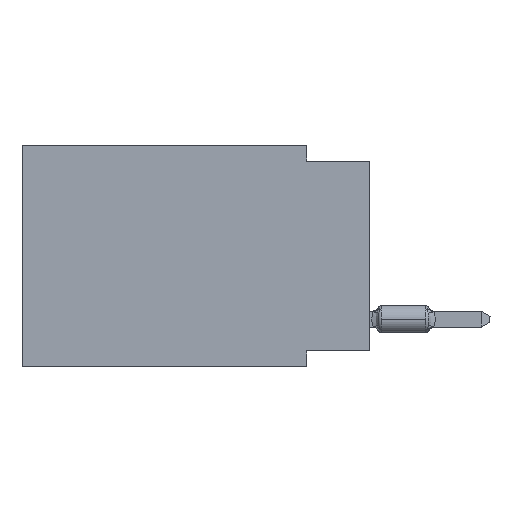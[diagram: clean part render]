
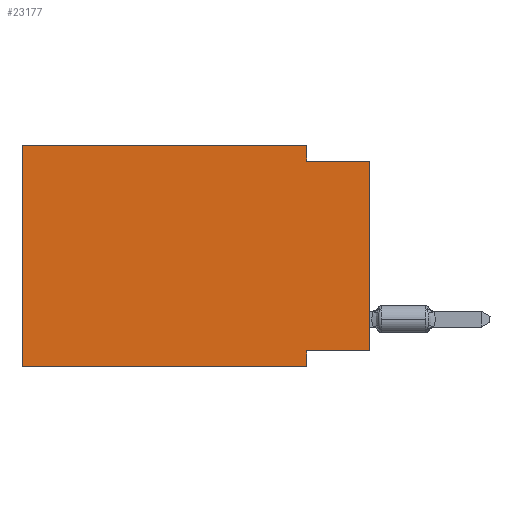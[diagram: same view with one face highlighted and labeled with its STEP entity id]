
A CAD part, left-side view. The second image highlights one B-rep face of the part: STEP entity #23177.
In plain terms, the highlighted planar face has unit normal (-1, 0, 0).
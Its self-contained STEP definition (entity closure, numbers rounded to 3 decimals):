
#3255 = DIRECTION ( 'NONE',  ( 1., 0., 0. ) ) ;
#3446 = VECTOR ( 'NONE', #14922, 1000. ) ;
#4065 = VERTEX_POINT ( 'NONE', #30810 ) ;
#4188 = VERTEX_POINT ( 'NONE', #8669 ) ;
#4518 = EDGE_CURVE ( 'NONE', #20491, #4188, #23478, .T. ) ;
#4533 = ORIENTED_EDGE ( 'NONE', *, *, #8984, .F. ) ;
#5095 = CARTESIAN_POINT ( 'NONE',  ( 0., 2.54, 0. ) ) ;
#5381 = CARTESIAN_POINT ( 'NONE',  ( 0., 13.97, 0. ) ) ;
#5508 = EDGE_CURVE ( 'NONE', #20491, #24755, #15888, .T. ) ;
#6417 = ORIENTED_EDGE ( 'NONE', *, *, #20811, .F. ) ;
#6539 = LINE ( 'NONE', #8978, #17832 ) ;
#6887 = ORIENTED_EDGE ( 'NONE', *, *, #11099, .T. ) ;
#6951 = EDGE_CURVE ( 'NONE', #24755, #10226, #9749, .T. ) ;
#7916 = EDGE_LOOP ( 'NONE', ( #22343, #30925, #11296, #4533, #6417, #6887, #31349, #20226 ) ) ;
#8182 = VECTOR ( 'NONE', #29321, 1000. ) ;
#8552 = VECTOR ( 'NONE', #33513, 1000. ) ;
#8659 = PLANE ( 'NONE',  #29451 ) ;
#8669 = CARTESIAN_POINT ( 'NONE',  ( 0., 0., -0.635 ) ) ;
#8978 = CARTESIAN_POINT ( 'NONE',  ( 0., 13.97, 0. ) ) ;
#8984 = EDGE_CURVE ( 'NONE', #32843, #20707, #32908, .T. ) ;
#9140 = EDGE_CURVE ( 'NONE', #4065, #4188, #30639, .T. ) ;
#9142 = VECTOR ( 'NONE', #15730, 1000. ) ;
#9749 = LINE ( 'NONE', #17945, #20324 ) ;
#10226 = VERTEX_POINT ( 'NONE', #16858 ) ;
#11099 = EDGE_CURVE ( 'NONE', #18466, #10226, #22703, .T. ) ;
#11296 = ORIENTED_EDGE ( 'NONE', *, *, #29015, .F. ) ;
#12833 = DIRECTION ( 'NONE',  ( 0., 0., 1. ) ) ;
#13177 = CARTESIAN_POINT ( 'NONE',  ( 0., 13.97, -8.89 ) ) ;
#13541 = CARTESIAN_POINT ( 'NONE',  ( 0., 2.54, 0. ) ) ;
#14564 = DIRECTION ( 'NONE',  ( 0., 0., 1. ) ) ;
#14922 = DIRECTION ( 'NONE',  ( 0., -1., 0. ) ) ;
#15149 = VECTOR ( 'NONE', #18788, 1000. ) ;
#15282 = CARTESIAN_POINT ( 'NONE',  ( 0., 0., 0. ) ) ;
#15730 = DIRECTION ( 'NONE',  ( 0., 0., -1. ) ) ;
#15888 = LINE ( 'NONE', #21978, #8182 ) ;
#16858 = CARTESIAN_POINT ( 'NONE',  ( 0., 2.54, -8.89 ) ) ;
#17832 = VECTOR ( 'NONE', #14564, 1000. ) ;
#17945 = CARTESIAN_POINT ( 'NONE',  ( 0., 2.54, -8.89 ) ) ;
#18466 = VERTEX_POINT ( 'NONE', #13177 ) ;
#18788 = DIRECTION ( 'NONE',  ( 0., -1., 0. ) ) ;
#20226 = ORIENTED_EDGE ( 'NONE', *, *, #5508, .F. ) ;
#20324 = VECTOR ( 'NONE', #26322, 1000. ) ;
#20491 = VERTEX_POINT ( 'NONE', #28205 ) ;
#20707 = VERTEX_POINT ( 'NONE', #13541 ) ;
#20811 = EDGE_CURVE ( 'NONE', #18466, #32843, #6539, .T. ) ;
#21978 = CARTESIAN_POINT ( 'NONE',  ( 0., 0., -8.255 ) ) ;
#22343 = ORIENTED_EDGE ( 'NONE', *, *, #4518, .T. ) ;
#22703 = LINE ( 'NONE', #30901, #8552 ) ;
#23177 = ADVANCED_FACE ( 'NONE', ( #32569 ), #8659, .F. ) ;
#23478 = LINE ( 'NONE', #15282, #26474 ) ;
#23912 = CARTESIAN_POINT ( 'NONE',  ( 0., 2.54, -8.255 ) ) ;
#24287 = LINE ( 'NONE', #5095, #9142 ) ;
#24755 = VERTEX_POINT ( 'NONE', #23912 ) ;
#26322 = DIRECTION ( 'NONE',  ( 0., 0., -1. ) ) ;
#26474 = VECTOR ( 'NONE', #12833, 1000. ) ;
#27169 = CARTESIAN_POINT ( 'NONE',  ( 0., 13.97, 0. ) ) ;
#27679 = CARTESIAN_POINT ( 'NONE',  ( 0., 0., -0.635 ) ) ;
#28205 = CARTESIAN_POINT ( 'NONE',  ( 0., 0., -8.255 ) ) ;
#29015 = EDGE_CURVE ( 'NONE', #20707, #4065, #24287, .T. ) ;
#29321 = DIRECTION ( 'NONE',  ( 0., 1., 0. ) ) ;
#29451 = AXIS2_PLACEMENT_3D ( 'NONE', #34515, #3255, #29940 ) ;
#29940 = DIRECTION ( 'NONE',  ( 0., 0., -1. ) ) ;
#30639 = LINE ( 'NONE', #27679, #3446 ) ;
#30810 = CARTESIAN_POINT ( 'NONE',  ( 0., 2.54, -0.635 ) ) ;
#30901 = CARTESIAN_POINT ( 'NONE',  ( 0., 13.97, -8.89 ) ) ;
#30925 = ORIENTED_EDGE ( 'NONE', *, *, #9140, .F. ) ;
#31349 = ORIENTED_EDGE ( 'NONE', *, *, #6951, .F. ) ;
#32569 = FACE_OUTER_BOUND ( 'NONE', #7916, .T. ) ;
#32843 = VERTEX_POINT ( 'NONE', #5381 ) ;
#32908 = LINE ( 'NONE', #27169, #15149 ) ;
#33513 = DIRECTION ( 'NONE',  ( 0., -1., 0. ) ) ;
#34515 = CARTESIAN_POINT ( 'NONE',  ( 0., 13.97, 0. ) ) ;
